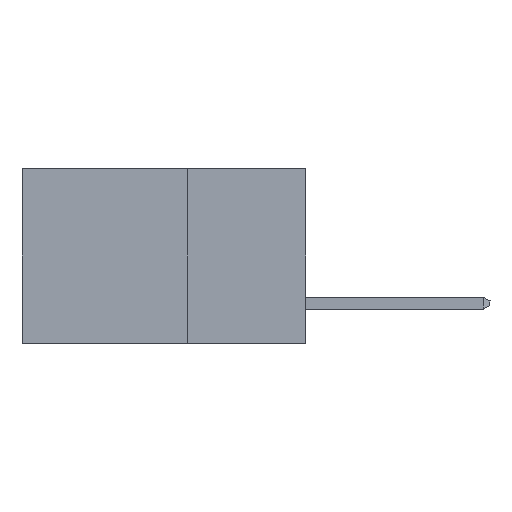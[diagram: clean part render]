
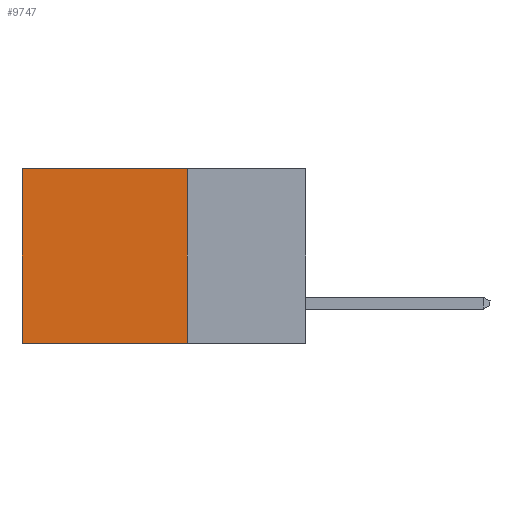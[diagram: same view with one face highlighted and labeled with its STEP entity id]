
A CAD part, left-side view. The second image highlights one B-rep face of the part: STEP entity #9747.
In plain terms, the highlighted planar face has unit normal (-1, 0, 0).
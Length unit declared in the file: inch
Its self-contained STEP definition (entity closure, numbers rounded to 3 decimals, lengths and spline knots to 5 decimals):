
#60 = ORIENTED_EDGE ( 'NONE', *, *, #892, .T. ) ;
#892 = EDGE_CURVE ( 'NONE', #3437, #8513, #1916, .T. ) ;
#1437 = LINE ( 'NONE', #9342, #14202 ) ;
#1916 = LINE ( 'NONE', #8380, #8007 ) ;
#2065 = CARTESIAN_POINT ( 'NONE',  ( 0.298, 0.6, 0. ) ) ;
#2204 = DIRECTION ( 'NONE',  ( 0., 0., -1. ) ) ;
#2228 = VERTEX_POINT ( 'NONE', #14967 ) ;
#2306 = DIRECTION ( 'NONE',  ( 0., 1., 0. ) ) ;
#2854 = ORIENTED_EDGE ( 'NONE', *, *, #6666, .F. ) ;
#3426 = VECTOR ( 'NONE', #10960, 39.37008 ) ;
#3437 = VERTEX_POINT ( 'NONE', #4845 ) ;
#4262 = LINE ( 'NONE', #2065, #13313 ) ;
#4497 = AXIS2_PLACEMENT_3D ( 'NONE', #11618, #11671, #2204 ) ;
#4626 = EDGE_CURVE ( 'NONE', #2228, #7556, #1437, .T. ) ;
#4798 = FACE_OUTER_BOUND ( 'NONE', #5222, .T. ) ;
#4845 = CARTESIAN_POINT ( 'NONE',  ( 0.298, 0.25, 0. ) ) ;
#5222 = EDGE_LOOP ( 'NONE', ( #8222, #7060, #2854, #60 ) ) ;
#6666 = EDGE_CURVE ( 'NONE', #3437, #2228, #9697, .T. ) ;
#7060 = ORIENTED_EDGE ( 'NONE', *, *, #4626, .F. ) ;
#7556 = VERTEX_POINT ( 'NONE', #9441 ) ;
#8007 = VECTOR ( 'NONE', #13273, 39.37008 ) ;
#8222 = ORIENTED_EDGE ( 'NONE', *, *, #9394, .T. ) ;
#8380 = CARTESIAN_POINT ( 'NONE',  ( 0.298, 0.25, 0. ) ) ;
#8513 = VERTEX_POINT ( 'NONE', #8599 ) ;
#8599 = CARTESIAN_POINT ( 'NONE',  ( 0.298, 0.6, 0. ) ) ;
#9068 = DIRECTION ( 'NONE',  ( 0., 0., -1. ) ) ;
#9342 = CARTESIAN_POINT ( 'NONE',  ( 0.298, 0.25, -0.37 ) ) ;
#9394 = EDGE_CURVE ( 'NONE', #8513, #7556, #4262, .T. ) ;
#9441 = CARTESIAN_POINT ( 'NONE',  ( 0.298, 0.6, -0.37 ) ) ;
#9697 = LINE ( 'NONE', #13560, #3426 ) ;
#9747 = ADVANCED_FACE ( 'NONE', ( #4798 ), #11463, .F. ) ;
#10960 = DIRECTION ( 'NONE',  ( 0., 0., -1. ) ) ;
#11463 = PLANE ( 'NONE',  #4497 ) ;
#11618 = CARTESIAN_POINT ( 'NONE',  ( 0.298, 0.25, 0. ) ) ;
#11671 = DIRECTION ( 'NONE',  ( 1., 0., 0. ) ) ;
#13273 = DIRECTION ( 'NONE',  ( 0., 1., 0. ) ) ;
#13313 = VECTOR ( 'NONE', #9068, 39.37008 ) ;
#13560 = CARTESIAN_POINT ( 'NONE',  ( 0.298, 0.25, 0. ) ) ;
#14202 = VECTOR ( 'NONE', #2306, 39.37008 ) ;
#14967 = CARTESIAN_POINT ( 'NONE',  ( 0.298, 0.25, -0.37 ) ) ;
